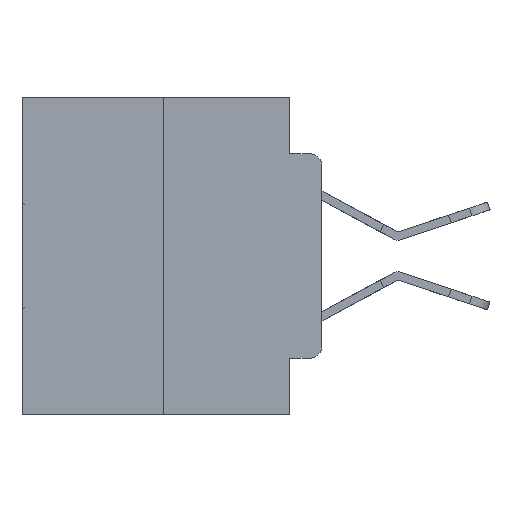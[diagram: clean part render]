
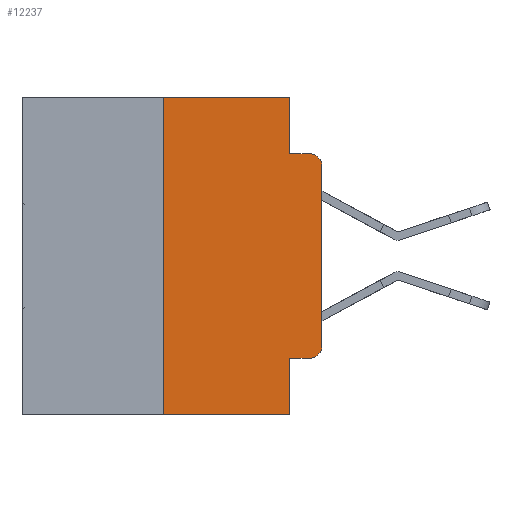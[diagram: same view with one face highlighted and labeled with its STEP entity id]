
A CAD part, left-side view. The second image highlights one B-rep face of the part: STEP entity #12237.
In plain terms, the highlighted planar face has unit normal (-1, 0, 0).
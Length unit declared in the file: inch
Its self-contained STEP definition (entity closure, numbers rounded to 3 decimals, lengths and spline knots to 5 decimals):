
#517 = VECTOR ( 'NONE', #16374, 39.37008 ) ;
#1038 = ORIENTED_EDGE ( 'NONE', *, *, #6612, .F. ) ;
#1392 = EDGE_CURVE ( 'NONE', #14926, #13602, #10274, .T. ) ;
#1675 = VECTOR ( 'NONE', #14790, 39.37008 ) ;
#1811 = ORIENTED_EDGE ( 'NONE', *, *, #25391, .F. ) ;
#2846 = LINE ( 'NONE', #8755, #8449 ) ;
#3005 = LINE ( 'NONE', #23130, #26265 ) ;
#4970 = DIRECTION ( 'NONE',  ( -1., 0., 0. ) ) ;
#5300 = EDGE_CURVE ( 'NONE', #28752, #13459, #28281, .T. ) ;
#5836 = LINE ( 'NONE', #29401, #6577 ) ;
#5851 = AXIS2_PLACEMENT_3D ( 'NONE', #6927, #23108, #9325 ) ;
#5956 = ORIENTED_EDGE ( 'NONE', *, *, #11167, .F. ) ;
#6577 = VECTOR ( 'NONE', #13364, 39.37008 ) ;
#6612 = EDGE_CURVE ( 'NONE', #24046, #28830, #18115, .T. ) ;
#6927 = CARTESIAN_POINT ( 'NONE',  ( 0., 0.02, -0.1085 ) ) ;
#6936 = AXIS2_PLACEMENT_3D ( 'NONE', #27937, #4970, #27836 ) ;
#7750 = CARTESIAN_POINT ( 'NONE',  ( 0., 0.051, 0. ) ) ;
#7998 = VECTOR ( 'NONE', #22089, 39.37008 ) ;
#8059 = FACE_OUTER_BOUND ( 'NONE', #18695, .T. ) ;
#8199 = ORIENTED_EDGE ( 'NONE', *, *, #5300, .T. ) ;
#8449 = VECTOR ( 'NONE', #29461, 39.37008 ) ;
#8755 = CARTESIAN_POINT ( 'NONE',  ( 0., 0., 0. ) ) ;
#8770 = EDGE_CURVE ( 'NONE', #15095, #24046, #3005, .T. ) ;
#8946 = ORIENTED_EDGE ( 'NONE', *, *, #25597, .F. ) ;
#9140 = CARTESIAN_POINT ( 'NONE',  ( 0., 0., -0.1085 ) ) ;
#9193 = CARTESIAN_POINT ( 'NONE',  ( 0., 0.25, 0. ) ) ;
#9199 = LINE ( 'NONE', #27827, #517 ) ;
#9325 = DIRECTION ( 'NONE',  ( 0., 0., -1. ) ) ;
#9672 = ORIENTED_EDGE ( 'NONE', *, *, #1392, .T. ) ;
#9694 = CARTESIAN_POINT ( 'NONE',  ( 0., 0.02, -0.0885 ) ) ;
#9999 = CARTESIAN_POINT ( 'NONE',  ( 0., 0., -0.3915 ) ) ;
#10274 = CIRCLE ( 'NONE', #6936, 0.02 ) ;
#10650 = VERTEX_POINT ( 'NONE', #9140 ) ;
#10765 = ORIENTED_EDGE ( 'NONE', *, *, #11970, .T. ) ;
#10916 = AXIS2_PLACEMENT_3D ( 'NONE', #19005, #25952, #12200 ) ;
#11167 = EDGE_CURVE ( 'NONE', #28830, #27026, #5836, .T. ) ;
#11315 = CARTESIAN_POINT ( 'NONE',  ( 0., 0.051, -0.0885 ) ) ;
#11970 = EDGE_CURVE ( 'NONE', #13602, #10650, #2846, .T. ) ;
#12104 = PLANE ( 'NONE',  #10916 ) ;
#12200 = DIRECTION ( 'NONE',  ( 0., 0., -1. ) ) ;
#12237 = ADVANCED_FACE ( 'NONE', ( #8059 ), #12104, .F. ) ;
#12749 = VECTOR ( 'NONE', #23296, 39.37008 ) ;
#13125 = EDGE_CURVE ( 'NONE', #15843, #14926, #21730, .T. ) ;
#13364 = DIRECTION ( 'NONE',  ( 0., -1., 0. ) ) ;
#13459 = VERTEX_POINT ( 'NONE', #27891 ) ;
#13602 = VERTEX_POINT ( 'NONE', #9999 ) ;
#13958 = CARTESIAN_POINT ( 'NONE',  ( 0., 0.051, 0. ) ) ;
#14315 = CARTESIAN_POINT ( 'NONE',  ( 0., 0.051, -0.4115 ) ) ;
#14790 = DIRECTION ( 'NONE',  ( 0., 0., -1. ) ) ;
#14926 = VERTEX_POINT ( 'NONE', #19756 ) ;
#15095 = VERTEX_POINT ( 'NONE', #9193 ) ;
#15535 = CIRCLE ( 'NONE', #5851, 0.02 ) ;
#15843 = VERTEX_POINT ( 'NONE', #14315 ) ;
#16060 = VECTOR ( 'NONE', #18631, 39.37008 ) ;
#16362 = EDGE_CURVE ( 'NONE', #10650, #27026, #15535, .T. ) ;
#16374 = DIRECTION ( 'NONE',  ( 0., 0., 1. ) ) ;
#16397 = LINE ( 'NONE', #7750, #1675 ) ;
#18115 = LINE ( 'NONE', #20993, #12749 ) ;
#18631 = DIRECTION ( 'NONE',  ( 0., -1., 0. ) ) ;
#18695 = EDGE_LOOP ( 'NONE', ( #10765, #23698, #5956, #1038, #25866, #1811, #8199, #8946, #27321, #9672 ) ) ;
#19005 = CARTESIAN_POINT ( 'NONE',  ( 0., 0.473, 0. ) ) ;
#19756 = CARTESIAN_POINT ( 'NONE',  ( 0., 0.02, -0.4115 ) ) ;
#20950 = CARTESIAN_POINT ( 'NONE',  ( 0., 0.473, -0.5 ) ) ;
#20993 = CARTESIAN_POINT ( 'NONE',  ( 0., 0.051, 0. ) ) ;
#21730 = LINE ( 'NONE', #26724, #7998 ) ;
#22089 = DIRECTION ( 'NONE',  ( 0., -1., 0. ) ) ;
#23108 = DIRECTION ( 'NONE',  ( -1., 0., 0. ) ) ;
#23130 = CARTESIAN_POINT ( 'NONE',  ( 0., 0.473, 0. ) ) ;
#23296 = DIRECTION ( 'NONE',  ( 0., 0., -1. ) ) ;
#23698 = ORIENTED_EDGE ( 'NONE', *, *, #16362, .T. ) ;
#24046 = VERTEX_POINT ( 'NONE', #13958 ) ;
#25391 = EDGE_CURVE ( 'NONE', #28752, #15095, #9199, .T. ) ;
#25430 = DIRECTION ( 'NONE',  ( 0., -1., 0. ) ) ;
#25597 = EDGE_CURVE ( 'NONE', #15843, #13459, #16397, .T. ) ;
#25866 = ORIENTED_EDGE ( 'NONE', *, *, #8770, .F. ) ;
#25952 = DIRECTION ( 'NONE',  ( 1., 0., 0. ) ) ;
#26265 = VECTOR ( 'NONE', #25430, 39.37008 ) ;
#26724 = CARTESIAN_POINT ( 'NONE',  ( 0., 0.051, -0.4115 ) ) ;
#27026 = VERTEX_POINT ( 'NONE', #9694 ) ;
#27321 = ORIENTED_EDGE ( 'NONE', *, *, #13125, .T. ) ;
#27827 = CARTESIAN_POINT ( 'NONE',  ( 0., 0.25, 0. ) ) ;
#27836 = DIRECTION ( 'NONE',  ( 0., 0., -1. ) ) ;
#27891 = CARTESIAN_POINT ( 'NONE',  ( 0., 0.051, -0.5 ) ) ;
#27937 = CARTESIAN_POINT ( 'NONE',  ( 0., 0.02, -0.3915 ) ) ;
#28281 = LINE ( 'NONE', #20950, #16060 ) ;
#28752 = VERTEX_POINT ( 'NONE', #29876 ) ;
#28830 = VERTEX_POINT ( 'NONE', #11315 ) ;
#29401 = CARTESIAN_POINT ( 'NONE',  ( 0., 0.051, -0.0885 ) ) ;
#29461 = DIRECTION ( 'NONE',  ( 0., 0., 1. ) ) ;
#29876 = CARTESIAN_POINT ( 'NONE',  ( 0., 0.25, -0.5 ) ) ;
